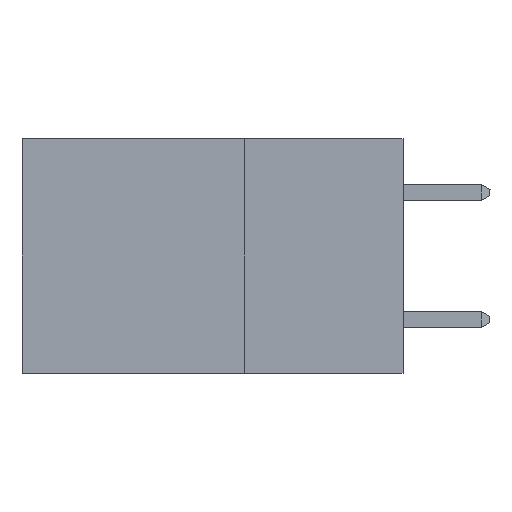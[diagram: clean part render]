
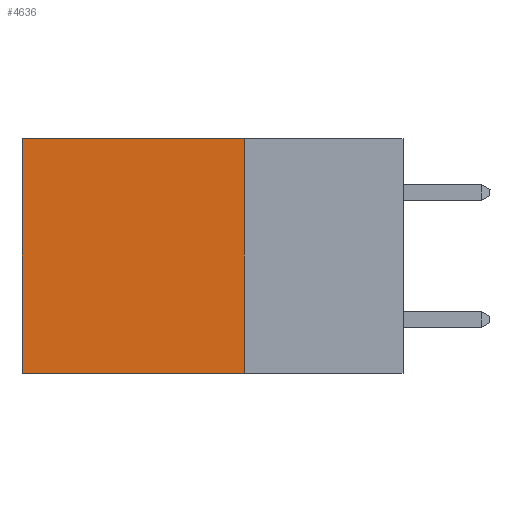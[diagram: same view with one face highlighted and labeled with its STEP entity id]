
A CAD part, left-side view. The second image highlights one B-rep face of the part: STEP entity #4636.
In plain terms, the highlighted planar face has unit normal (-1, 0, 0).
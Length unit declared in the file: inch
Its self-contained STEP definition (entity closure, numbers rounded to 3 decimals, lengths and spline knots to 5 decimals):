
#46 = CARTESIAN_POINT ( 'NONE',  ( 0.2875, 0.25, -0.37 ) ) ;
#75 = FACE_OUTER_BOUND ( 'NONE', #9855, .T. ) ;
#140 = DIRECTION ( 'NONE',  ( 1., 0., 0. ) ) ;
#258 = ORIENTED_EDGE ( 'NONE', *, *, #1298, .F. ) ;
#274 = LINE ( 'NONE', #8033, #5802 ) ;
#761 = EDGE_CURVE ( 'NONE', #7073, #9780, #9061, .T. ) ;
#822 = CARTESIAN_POINT ( 'NONE',  ( 0.2875, 0.6, -0.37 ) ) ;
#939 = DIRECTION ( 'NONE',  ( 0., 1., 0. ) ) ;
#1206 = VERTEX_POINT ( 'NONE', #8198 ) ;
#1207 = ORIENTED_EDGE ( 'NONE', *, *, #8845, .T. ) ;
#1298 = EDGE_CURVE ( 'NONE', #4265, #7073, #4694, .T. ) ;
#1309 = CARTESIAN_POINT ( 'NONE',  ( 0.2875, 0.25, 0. ) ) ;
#1809 = ORIENTED_EDGE ( 'NONE', *, *, #761, .F. ) ;
#2469 = VECTOR ( 'NONE', #8251, 39.37008 ) ;
#4014 = PLANE ( 'NONE',  #7166 ) ;
#4162 = LINE ( 'NONE', #7838, #4542 ) ;
#4265 = VERTEX_POINT ( 'NONE', #4363 ) ;
#4363 = CARTESIAN_POINT ( 'NONE',  ( 0.2875, 0.25, 0. ) ) ;
#4542 = VECTOR ( 'NONE', #5346, 39.37008 ) ;
#4636 = ADVANCED_FACE ( 'NONE', ( #75 ), #4014, .F. ) ;
#4694 = LINE ( 'NONE', #1309, #2469 ) ;
#4849 = DIRECTION ( 'NONE',  ( 0., 0., -1. ) ) ;
#5346 = DIRECTION ( 'NONE',  ( 0., 1., 0. ) ) ;
#5617 = CARTESIAN_POINT ( 'NONE',  ( 0.2875, 0.25, -0.37 ) ) ;
#5802 = VECTOR ( 'NONE', #8108, 39.37008 ) ;
#7073 = VERTEX_POINT ( 'NONE', #5617 ) ;
#7092 = EDGE_CURVE ( 'NONE', #1206, #9780, #274, .T. ) ;
#7166 = AXIS2_PLACEMENT_3D ( 'NONE', #8898, #140, #4849 ) ;
#7838 = CARTESIAN_POINT ( 'NONE',  ( 0.2875, 0.25, 0. ) ) ;
#8033 = CARTESIAN_POINT ( 'NONE',  ( 0.2875, 0.6, 0. ) ) ;
#8108 = DIRECTION ( 'NONE',  ( 0., 0., -1. ) ) ;
#8124 = ORIENTED_EDGE ( 'NONE', *, *, #7092, .T. ) ;
#8198 = CARTESIAN_POINT ( 'NONE',  ( 0.2875, 0.6, 0. ) ) ;
#8251 = DIRECTION ( 'NONE',  ( 0., 0., -1. ) ) ;
#8804 = VECTOR ( 'NONE', #939, 39.37008 ) ;
#8845 = EDGE_CURVE ( 'NONE', #4265, #1206, #4162, .T. ) ;
#8898 = CARTESIAN_POINT ( 'NONE',  ( 0.2875, 0.25, 0. ) ) ;
#9061 = LINE ( 'NONE', #46, #8804 ) ;
#9780 = VERTEX_POINT ( 'NONE', #822 ) ;
#9855 = EDGE_LOOP ( 'NONE', ( #8124, #1809, #258, #1207 ) ) ;
